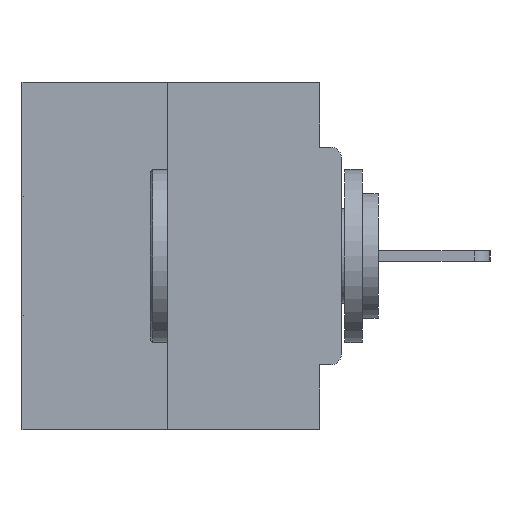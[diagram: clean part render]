
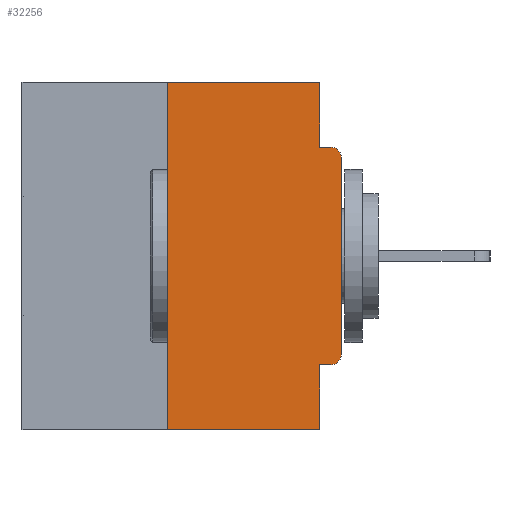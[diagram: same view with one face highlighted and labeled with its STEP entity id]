
A CAD part, left-side view. The second image highlights one B-rep face of the part: STEP entity #32256.
In plain terms, the highlighted planar face has unit normal (-1, 0, 0).
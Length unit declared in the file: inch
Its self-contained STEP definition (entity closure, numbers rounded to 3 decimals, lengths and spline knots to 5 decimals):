
#1110 = FACE_OUTER_BOUND ( 'NONE', #13039, .T. ) ;
#1315 = VERTEX_POINT ( 'NONE', #9062 ) ;
#1770 = ORIENTED_EDGE ( 'NONE', *, *, #31439, .F. ) ;
#1963 = DIRECTION ( 'NONE',  ( 0., 0., -1. ) ) ;
#2020 = CARTESIAN_POINT ( 'NONE',  ( 0., 0., -0.0935 ) ) ;
#2068 = LINE ( 'NONE', #23557, #33926 ) ;
#2127 = EDGE_CURVE ( 'NONE', #4630, #23499, #23563, .T. ) ;
#2731 = VECTOR ( 'NONE', #16854, 39.37008 ) ;
#2741 = ORIENTED_EDGE ( 'NONE', *, *, #23046, .F. ) ;
#2892 = CARTESIAN_POINT ( 'NONE',  ( 0., 0.015, -0.3915 ) ) ;
#3223 = DIRECTION ( 'NONE',  ( 0., 0., -1. ) ) ;
#3244 = ORIENTED_EDGE ( 'NONE', *, *, #10917, .F. ) ;
#3926 = VERTEX_POINT ( 'NONE', #30964 ) ;
#4042 = CARTESIAN_POINT ( 'NONE',  ( 0., 0.25, -0.5 ) ) ;
#4076 = ORIENTED_EDGE ( 'NONE', *, *, #4917, .F. ) ;
#4630 = VERTEX_POINT ( 'NONE', #32955 ) ;
#4857 = DIRECTION ( 'NONE',  ( 0., 0., -1. ) ) ;
#4917 = EDGE_CURVE ( 'NONE', #32500, #3926, #21241, .T. ) ;
#5605 = CARTESIAN_POINT ( 'NONE',  ( 0., 0.031, -0.5 ) ) ;
#5654 = CARTESIAN_POINT ( 'NONE',  ( 0., 0.031, -0.4065 ) ) ;
#6028 = EDGE_CURVE ( 'NONE', #23499, #21283, #19358, .T. ) ;
#6540 = DIRECTION ( 'NONE',  ( 1., 0., 0. ) ) ;
#8273 = AXIS2_PLACEMENT_3D ( 'NONE', #19799, #6540, #14200 ) ;
#8278 = CIRCLE ( 'NONE', #33957, 0.015 ) ;
#8842 = LINE ( 'NONE', #27367, #2731 ) ;
#9062 = CARTESIAN_POINT ( 'NONE',  ( 0., 0.015, -0.0935 ) ) ;
#10917 = EDGE_CURVE ( 'NONE', #27932, #24090, #29324, .T. ) ;
#11329 = CARTESIAN_POINT ( 'NONE',  ( 0., 0., 0. ) ) ;
#11780 = PLANE ( 'NONE',  #8273 ) ;
#12653 = DIRECTION ( 'NONE',  ( 0., 0., 1. ) ) ;
#12814 = CARTESIAN_POINT ( 'NONE',  ( 0., 0.25, 0. ) ) ;
#13039 = EDGE_LOOP ( 'NONE', ( #32718, #21234, #25304, #3244, #1770, #34142, #22035, #26607, #2741, #4076 ) ) ;
#14200 = DIRECTION ( 'NONE',  ( 0., 0., -1. ) ) ;
#15279 = LINE ( 'NONE', #2020, #18908 ) ;
#15511 = DIRECTION ( 'NONE',  ( 0., 1., 0. ) ) ;
#15706 = CARTESIAN_POINT ( 'NONE',  ( 0., 0.46, 0. ) ) ;
#15967 = CARTESIAN_POINT ( 'NONE',  ( 0., 0.031, 0. ) ) ;
#16854 = DIRECTION ( 'NONE',  ( 0., -1., 0. ) ) ;
#17944 = CARTESIAN_POINT ( 'NONE',  ( 0., 0.031, -0.5 ) ) ;
#18375 = DIRECTION ( 'NONE',  ( -1., 0., 0. ) ) ;
#18633 = VECTOR ( 'NONE', #29541, 39.37008 ) ;
#18908 = VECTOR ( 'NONE', #31374, 39.37008 ) ;
#18930 = VECTOR ( 'NONE', #12653, 39.37008 ) ;
#19260 = VERTEX_POINT ( 'NONE', #4042 ) ;
#19358 = LINE ( 'NONE', #11329, #18633 ) ;
#19365 = CARTESIAN_POINT ( 'NONE',  ( 0., 0.031, 0. ) ) ;
#19799 = CARTESIAN_POINT ( 'NONE',  ( 0., 0.46, 0. ) ) ;
#21146 = LINE ( 'NONE', #15706, #28489 ) ;
#21234 = ORIENTED_EDGE ( 'NONE', *, *, #33319, .F. ) ;
#21241 = LINE ( 'NONE', #15967, #31432 ) ;
#21283 = VERTEX_POINT ( 'NONE', #31243 ) ;
#22035 = ORIENTED_EDGE ( 'NONE', *, *, #6028, .T. ) ;
#22069 = EDGE_CURVE ( 'NONE', #21283, #1315, #8278, .T. ) ;
#22700 = EDGE_CURVE ( 'NONE', #19260, #24090, #8842, .T. ) ;
#22793 = LINE ( 'NONE', #33284, #18930 ) ;
#23046 = EDGE_CURVE ( 'NONE', #3926, #1315, #15279, .T. ) ;
#23499 = VERTEX_POINT ( 'NONE', #33955 ) ;
#23557 = CARTESIAN_POINT ( 'NONE',  ( 0., 0., -0.4065 ) ) ;
#23563 = CIRCLE ( 'NONE', #31375, 0.015 ) ;
#24090 = VERTEX_POINT ( 'NONE', #5605 ) ;
#25304 = ORIENTED_EDGE ( 'NONE', *, *, #22700, .T. ) ;
#26377 = DIRECTION ( 'NONE',  ( 0., -1., 0. ) ) ;
#26525 = VERTEX_POINT ( 'NONE', #12814 ) ;
#26607 = ORIENTED_EDGE ( 'NONE', *, *, #22069, .T. ) ;
#27367 = CARTESIAN_POINT ( 'NONE',  ( 0., 0.46, -0.5 ) ) ;
#27932 = VERTEX_POINT ( 'NONE', #5654 ) ;
#28489 = VECTOR ( 'NONE', #26377, 39.37008 ) ;
#28698 = CARTESIAN_POINT ( 'NONE',  ( 0., 0.015, -0.1085 ) ) ;
#29234 = VECTOR ( 'NONE', #4857, 39.37008 ) ;
#29324 = LINE ( 'NONE', #17944, #29234 ) ;
#29541 = DIRECTION ( 'NONE',  ( 0., 0., 1. ) ) ;
#30152 = DIRECTION ( 'NONE',  ( -1., 0., 0. ) ) ;
#30964 = CARTESIAN_POINT ( 'NONE',  ( 0., 0.031, -0.0935 ) ) ;
#31243 = CARTESIAN_POINT ( 'NONE',  ( 0., 0., -0.1085 ) ) ;
#31374 = DIRECTION ( 'NONE',  ( 0., -1., 0. ) ) ;
#31375 = AXIS2_PLACEMENT_3D ( 'NONE', #2892, #30152, #3223 ) ;
#31432 = VECTOR ( 'NONE', #31895, 39.37008 ) ;
#31439 = EDGE_CURVE ( 'NONE', #4630, #27932, #2068, .T. ) ;
#31895 = DIRECTION ( 'NONE',  ( 0., 0., -1. ) ) ;
#32256 = ADVANCED_FACE ( 'NONE', ( #1110 ), #11780, .F. ) ;
#32500 = VERTEX_POINT ( 'NONE', #19365 ) ;
#32718 = ORIENTED_EDGE ( 'NONE', *, *, #34305, .F. ) ;
#32955 = CARTESIAN_POINT ( 'NONE',  ( 0., 0.015, -0.4065 ) ) ;
#33284 = CARTESIAN_POINT ( 'NONE',  ( 0., 0.25, 0. ) ) ;
#33319 = EDGE_CURVE ( 'NONE', #19260, #26525, #22793, .T. ) ;
#33926 = VECTOR ( 'NONE', #15511, 39.37008 ) ;
#33955 = CARTESIAN_POINT ( 'NONE',  ( 0., 0., -0.3915 ) ) ;
#33957 = AXIS2_PLACEMENT_3D ( 'NONE', #28698, #18375, #1963 ) ;
#34142 = ORIENTED_EDGE ( 'NONE', *, *, #2127, .T. ) ;
#34305 = EDGE_CURVE ( 'NONE', #26525, #32500, #21146, .T. ) ;
